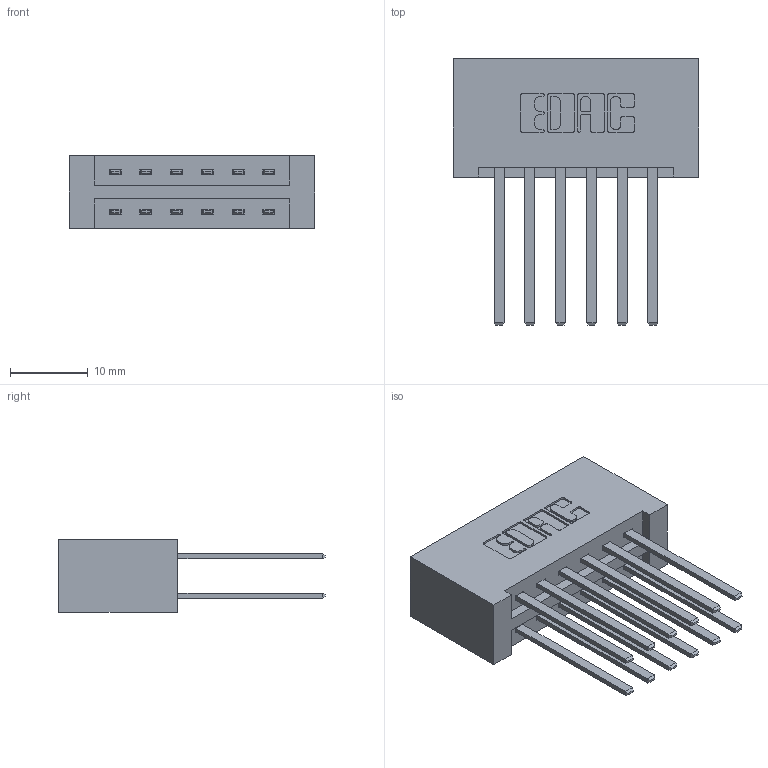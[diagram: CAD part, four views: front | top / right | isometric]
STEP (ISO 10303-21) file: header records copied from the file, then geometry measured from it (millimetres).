
FILE_DESCRIPTION (( 'STEP AP203' ), '1' );
FILE_NAME ('387-012-544-201.STEP', '2019-10-15T20:04:32', ( '' ), ( '' ), 'SwSTEP 2.0', 'SolidWorks 2016', '' );
FILE_SCHEMA (( 'CONFIG_CONTROL_DESIGN' ));
Length unit declared in the file: inch
Products named in the file (3): 345-292-001_345-293-144; 387-012-544-201; 337 Part_No Mounting Lugs
Assembly tree (13 placements, depth 2):
  387-012-544-201
    337 Part_No Mounting Lugs
    345-292-001_345-293-144  x12
Bounding box: 31.65 x 34.3 x 9.4 mm (x, y, z)
Volume: 3785.1 mm3; surface area: 4535 mm2
Topology: 13 solids, 13 shells, 682 faces, 2003 edges, 1318 vertices
Faces by surface type: plane 474, cylinder 208
Entity records: 8847 total; most frequent: CARTESIAN_POINT 1518, ORIENTED_EDGE 1454, DIRECTION 1347, EDGE_CURVE 727, LINE 611, VECTOR 611, VERTEX_POINT 482, AXIS2_PLACEMENT_3D 368
